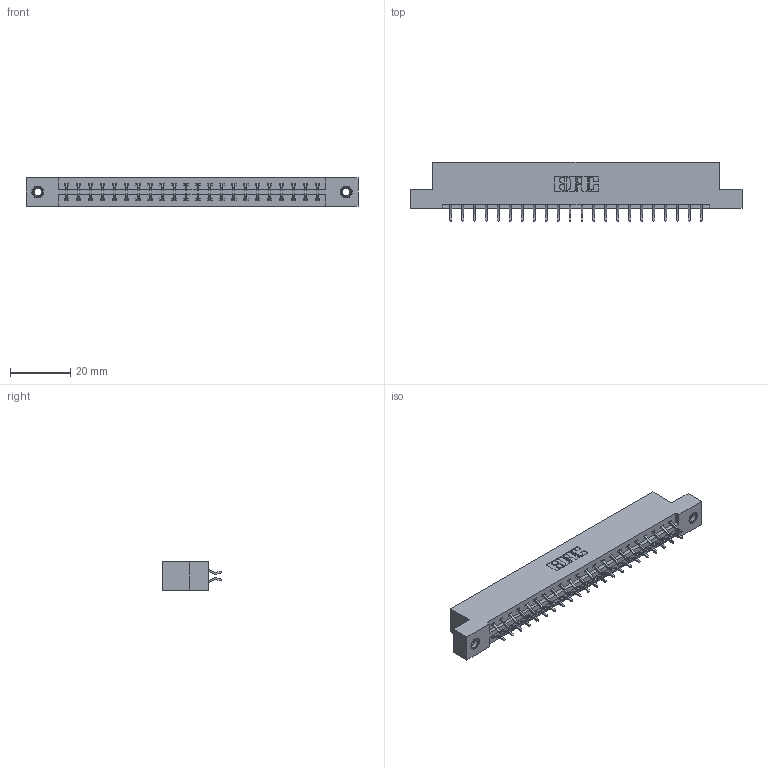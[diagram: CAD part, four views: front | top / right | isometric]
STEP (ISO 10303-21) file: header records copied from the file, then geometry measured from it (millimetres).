
FILE_DESCRIPTION (( 'STEP AP203' ), '1' );
FILE_NAME ('387-044-556-207.STEP', '2018-09-20T02:45:36', ( '' ), ( '' ), 'SwSTEP 2.0', 'SolidWorks 2016', '' );
FILE_SCHEMA (( 'CONFIG_CONTROL_DESIGN' ));
Length unit declared in the file: inch
Products named in the file (4): 337 Part_Flush Mounting Lugs - 0.156 Dia-TI; 345-292-001_556 Tail; 345-250-001_345-250-005-103; 387-044-556-207
Assembly tree (47 placements, depth 2):
  387-044-556-207
    337 Part_Flush Mounting Lugs - 0.156 Dia-TI
    345-292-001_556 Tail  x44
    345-250-001_345-250-005-103  x2
Bounding box: 110.19 x 19.57 x 9.4 mm (x, y, z)
Volume: 11330.7 mm3; surface area: 12604.6 mm2
Topology: 47 solids, 47 shells, 2814 faces, 8323 edges, 5482 vertices
Faces by surface type: plane 1950, cylinder 848, cone 12, torus 4
Entity records: 21050 total; most frequent: CARTESIAN_POINT 3557, ORIENTED_EDGE 3474, DIRECTION 3083, EDGE_CURVE 1737, VECTOR 1581, LINE 1581, VERTEX_POINT 1152, AXIS2_PLACEMENT_3D 751
